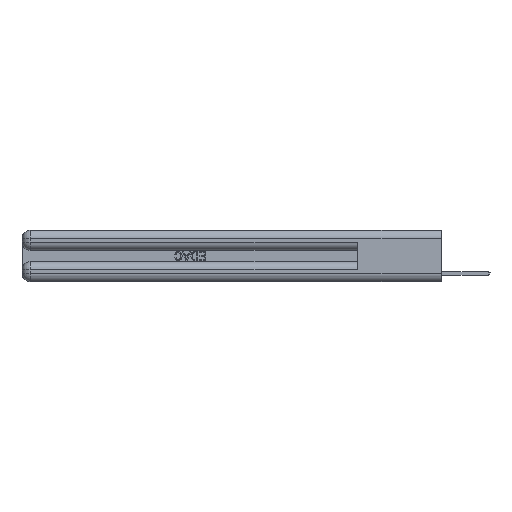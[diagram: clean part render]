
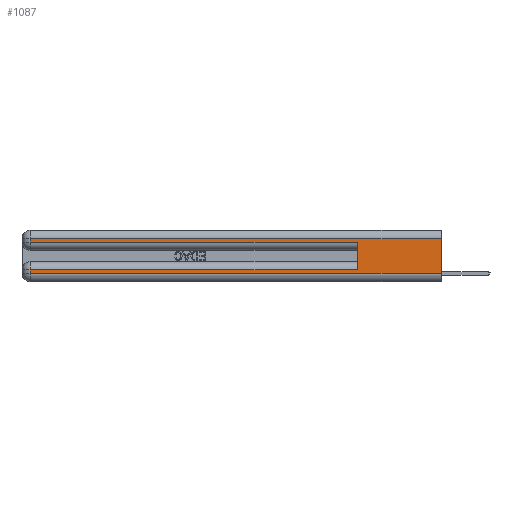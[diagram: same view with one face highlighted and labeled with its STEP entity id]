
A CAD part, left-side view. The second image highlights one B-rep face of the part: STEP entity #1087.
In plain terms, the highlighted planar face has unit normal (-1, 0, 0).
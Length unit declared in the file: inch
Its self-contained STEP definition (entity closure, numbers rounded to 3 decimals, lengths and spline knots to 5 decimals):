
#525 = DIRECTION ( 'NONE',  ( 1., 0., 0. ) ) ;
#1087 = ADVANCED_FACE ( 'NONE', ( #26130 ), #23841, .F. ) ;
#1638 = CARTESIAN_POINT ( 'NONE',  ( 0., 0., 0.285 ) ) ;
#1735 = ORIENTED_EDGE ( 'NONE', *, *, #4139, .T. ) ;
#1859 = CARTESIAN_POINT ( 'NONE',  ( 0., 0.6, 0.285 ) ) ;
#2341 = VECTOR ( 'NONE', #3499, 39.37008 ) ;
#2774 = CARTESIAN_POINT ( 'NONE',  ( 0., 0., 0.06 ) ) ;
#2823 = CARTESIAN_POINT ( 'NONE',  ( 0., 0., 0.37 ) ) ;
#3499 = DIRECTION ( 'NONE',  ( 0., 0., -1. ) ) ;
#4139 = EDGE_CURVE ( 'NONE', #27974, #4837, #22511, .T. ) ;
#4680 = LINE ( 'NONE', #8980, #12172 ) ;
#4837 = VERTEX_POINT ( 'NONE', #1859 ) ;
#5213 = VECTOR ( 'NONE', #9166, 39.37008 ) ;
#5540 = LINE ( 'NONE', #26220, #25287 ) ;
#6412 = CARTESIAN_POINT ( 'NONE',  ( 0., 0.6, 0.085 ) ) ;
#7043 = CARTESIAN_POINT ( 'NONE',  ( 0., 2.94, 0.285 ) ) ;
#7240 = ORIENTED_EDGE ( 'NONE', *, *, #28804, .F. ) ;
#7347 = VERTEX_POINT ( 'NONE', #9777 ) ;
#7433 = CARTESIAN_POINT ( 'NONE',  ( 0., 0., 0.06 ) ) ;
#7833 = EDGE_CURVE ( 'NONE', #10346, #4837, #5540, .T. ) ;
#8271 = EDGE_CURVE ( 'NONE', #16754, #21119, #14478, .T. ) ;
#8298 = ORIENTED_EDGE ( 'NONE', *, *, #17989, .T. ) ;
#8980 = CARTESIAN_POINT ( 'NONE',  ( 0., 0., 0.37 ) ) ;
#9166 = DIRECTION ( 'NONE',  ( 0., 1., 0. ) ) ;
#9777 = CARTESIAN_POINT ( 'NONE',  ( 0., 2.94, 0.085 ) ) ;
#9865 = DIRECTION ( 'NONE',  ( 0., -1., 0. ) ) ;
#10346 = VERTEX_POINT ( 'NONE', #6412 ) ;
#10802 = LINE ( 'NONE', #29584, #28788 ) ;
#10891 = DIRECTION ( 'NONE',  ( 0., -1., 0. ) ) ;
#12172 = VECTOR ( 'NONE', #14049, 39.37008 ) ;
#12928 = DIRECTION ( 'NONE',  ( 0., 0., -1. ) ) ;
#12961 = DIRECTION ( 'NONE',  ( 0., 1., 0. ) ) ;
#14049 = DIRECTION ( 'NONE',  ( 0., 0., -1. ) ) ;
#14082 = EDGE_LOOP ( 'NONE', ( #7240, #17883, #21430, #1735, #22120, #27552, #8298, #27858 ) ) ;
#14383 = EDGE_CURVE ( 'NONE', #10346, #7347, #20634, .T. ) ;
#14478 = LINE ( 'NONE', #2774, #29175 ) ;
#14765 = DIRECTION ( 'NONE',  ( 0., 0., 1. ) ) ;
#16754 = VERTEX_POINT ( 'NONE', #19607 ) ;
#17247 = CARTESIAN_POINT ( 'NONE',  ( 0., 2.94, 0.31 ) ) ;
#17334 = LINE ( 'NONE', #17481, #2341 ) ;
#17481 = CARTESIAN_POINT ( 'NONE',  ( 0., 2.94, 0.37 ) ) ;
#17883 = ORIENTED_EDGE ( 'NONE', *, *, #18446, .T. ) ;
#17989 = EDGE_CURVE ( 'NONE', #7347, #16754, #17334, .T. ) ;
#18136 = CARTESIAN_POINT ( 'NONE',  ( 0., 0., 0.31 ) ) ;
#18446 = EDGE_CURVE ( 'NONE', #18596, #28892, #10802, .T. ) ;
#18596 = VERTEX_POINT ( 'NONE', #18136 ) ;
#18870 = EDGE_CURVE ( 'NONE', #28892, #27974, #26690, .T. ) ;
#19231 = DIRECTION ( 'NONE',  ( 0., 0., -1. ) ) ;
#19607 = CARTESIAN_POINT ( 'NONE',  ( 0., 2.94, 0.06 ) ) ;
#20634 = LINE ( 'NONE', #29936, #5213 ) ;
#21119 = VERTEX_POINT ( 'NONE', #7433 ) ;
#21430 = ORIENTED_EDGE ( 'NONE', *, *, #18870, .T. ) ;
#22120 = ORIENTED_EDGE ( 'NONE', *, *, #7833, .F. ) ;
#22511 = LINE ( 'NONE', #1638, #26060 ) ;
#23841 = PLANE ( 'NONE',  #29412 ) ;
#25287 = VECTOR ( 'NONE', #14765, 39.37008 ) ;
#26060 = VECTOR ( 'NONE', #10891, 39.37008 ) ;
#26130 = FACE_OUTER_BOUND ( 'NONE', #14082, .T. ) ;
#26220 = CARTESIAN_POINT ( 'NONE',  ( 0., 0.6, 0.145 ) ) ;
#26690 = LINE ( 'NONE', #29250, #29749 ) ;
#27552 = ORIENTED_EDGE ( 'NONE', *, *, #14383, .T. ) ;
#27858 = ORIENTED_EDGE ( 'NONE', *, *, #8271, .T. ) ;
#27974 = VERTEX_POINT ( 'NONE', #7043 ) ;
#28788 = VECTOR ( 'NONE', #12961, 39.37008 ) ;
#28804 = EDGE_CURVE ( 'NONE', #18596, #21119, #4680, .T. ) ;
#28892 = VERTEX_POINT ( 'NONE', #17247 ) ;
#29175 = VECTOR ( 'NONE', #9865, 39.37008 ) ;
#29250 = CARTESIAN_POINT ( 'NONE',  ( 0., 2.94, 0.37 ) ) ;
#29412 = AXIS2_PLACEMENT_3D ( 'NONE', #2823, #525, #19231 ) ;
#29584 = CARTESIAN_POINT ( 'NONE',  ( 0., 0., 0.31 ) ) ;
#29749 = VECTOR ( 'NONE', #12928, 39.37008 ) ;
#29936 = CARTESIAN_POINT ( 'NONE',  ( 0., 0., 0.085 ) ) ;
